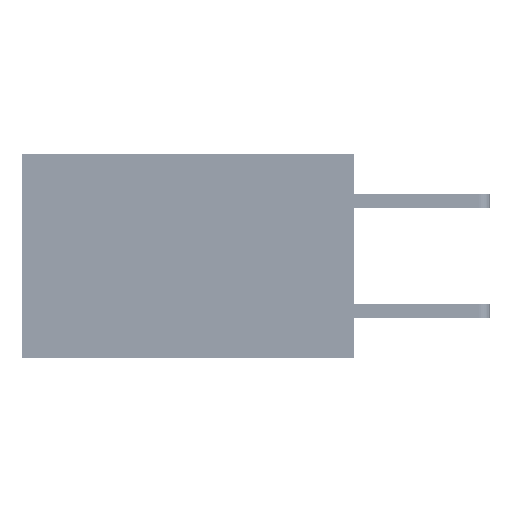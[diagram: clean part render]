
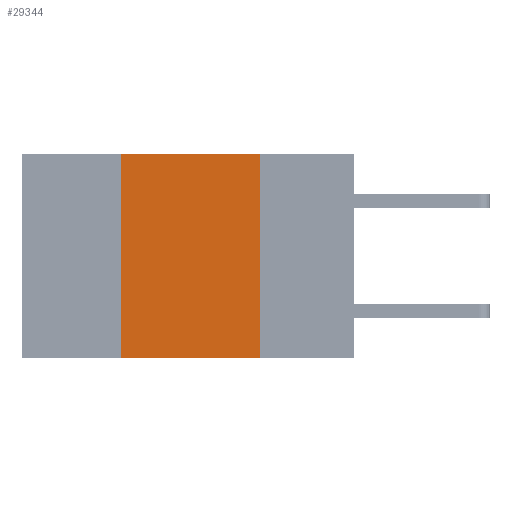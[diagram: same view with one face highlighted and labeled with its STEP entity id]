
A CAD part, left-side view. The second image highlights one B-rep face of the part: STEP entity #29344.
In plain terms, the highlighted planar face has unit normal (-1, 0, 0).
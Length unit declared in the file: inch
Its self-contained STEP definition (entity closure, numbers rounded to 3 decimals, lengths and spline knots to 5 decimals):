
#528 = CARTESIAN_POINT ( 'NONE',  ( 0., 0.17, 0. ) ) ;
#2567 = LINE ( 'NONE', #14203, #44641 ) ;
#3216 = FACE_OUTER_BOUND ( 'NONE', #6474, .T. ) ;
#3477 = DIRECTION ( 'NONE',  ( 0., -1., 0. ) ) ;
#5123 = ORIENTED_EDGE ( 'NONE', *, *, #33068, .T. ) ;
#5425 = VERTEX_POINT ( 'NONE', #38045 ) ;
#5948 = VERTEX_POINT ( 'NONE', #528 ) ;
#6011 = PLANE ( 'NONE',  #44646 ) ;
#6035 = ORIENTED_EDGE ( 'NONE', *, *, #25063, .F. ) ;
#6474 = EDGE_LOOP ( 'NONE', ( #9334, #6035, #24127, #5123 ) ) ;
#9334 = ORIENTED_EDGE ( 'NONE', *, *, #47658, .F. ) ;
#14203 = CARTESIAN_POINT ( 'NONE',  ( 0., 0.17, 0. ) ) ;
#14325 = DIRECTION ( 'NONE',  ( 1., 0., 0. ) ) ;
#16048 = CARTESIAN_POINT ( 'NONE',  ( 0., 0.6, 0. ) ) ;
#18598 = DIRECTION ( 'NONE',  ( 0., 0., -1. ) ) ;
#18660 = VERTEX_POINT ( 'NONE', #29579 ) ;
#19743 = LINE ( 'NONE', #35161, #44690 ) ;
#19967 = DIRECTION ( 'NONE',  ( 0., 0., 1. ) ) ;
#23623 = LINE ( 'NONE', #16048, #27581 ) ;
#24127 = ORIENTED_EDGE ( 'NONE', *, *, #24435, .F. ) ;
#24435 = EDGE_CURVE ( 'NONE', #5425, #18660, #19743, .T. ) ;
#25063 = EDGE_CURVE ( 'NONE', #18660, #5948, #23623, .T. ) ;
#27581 = VECTOR ( 'NONE', #3477, 39.37008 ) ;
#29344 = ADVANCED_FACE ( 'NONE', ( #3216 ), #6011, .F. ) ;
#29579 = CARTESIAN_POINT ( 'NONE',  ( 0., 0.42, 0. ) ) ;
#33068 = EDGE_CURVE ( 'NONE', #5425, #46758, #45696, .T. ) ;
#34124 = DIRECTION ( 'NONE',  ( 0., -1., 0. ) ) ;
#35161 = CARTESIAN_POINT ( 'NONE',  ( 0., 0.42, 0. ) ) ;
#37895 = CARTESIAN_POINT ( 'NONE',  ( 0., 0.6, -0.37 ) ) ;
#38045 = CARTESIAN_POINT ( 'NONE',  ( 0., 0.42, -0.37 ) ) ;
#39804 = CARTESIAN_POINT ( 'NONE',  ( 0., 0.17, -0.37 ) ) ;
#40393 = VECTOR ( 'NONE', #34124, 39.37008 ) ;
#40687 = DIRECTION ( 'NONE',  ( 0., 0., -1. ) ) ;
#44641 = VECTOR ( 'NONE', #40687, 39.37008 ) ;
#44646 = AXIS2_PLACEMENT_3D ( 'NONE', #48871, #14325, #18598 ) ;
#44690 = VECTOR ( 'NONE', #19967, 39.37008 ) ;
#45696 = LINE ( 'NONE', #37895, #40393 ) ;
#46758 = VERTEX_POINT ( 'NONE', #39804 ) ;
#47658 = EDGE_CURVE ( 'NONE', #5948, #46758, #2567, .T. ) ;
#48871 = CARTESIAN_POINT ( 'NONE',  ( 0., 0.6, 0. ) ) ;
